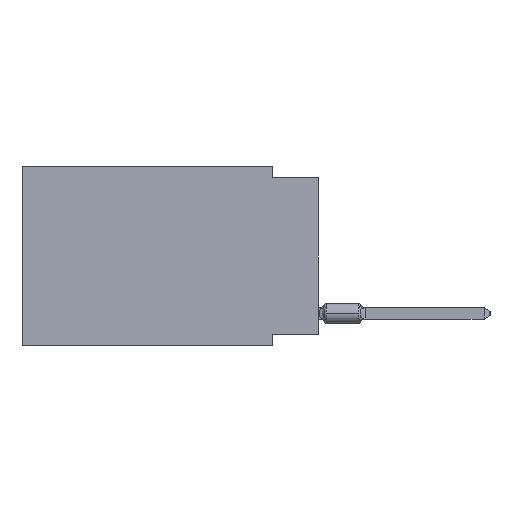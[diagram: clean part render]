
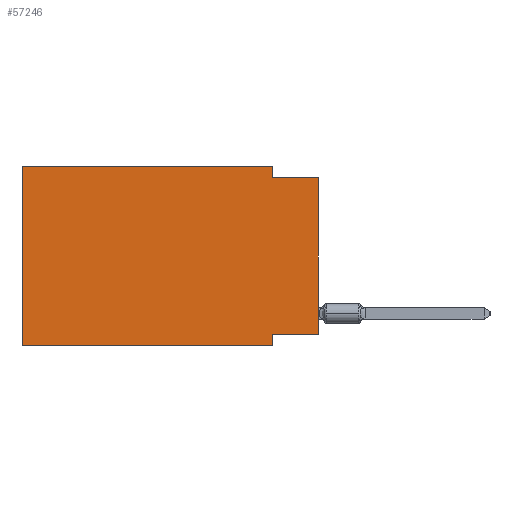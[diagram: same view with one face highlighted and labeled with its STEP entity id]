
A CAD part, left-side view. The second image highlights one B-rep face of the part: STEP entity #57246.
In plain terms, the highlighted planar face has unit normal (-1, 0, 0).
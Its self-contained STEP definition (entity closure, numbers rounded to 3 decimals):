
#86787 = CARTESIAN_POINT ( 'NONE',  ( 0., 0., -9.271 ) ) ;
#5160 = VERTEX_POINT ( 'NONE', #24850 ) ;
#6858 = VECTOR ( 'NONE', #38476, 1000. ) ;
#7060 = DIRECTION ( 'NONE',  ( 0., 0., 1. ) ) ;
#8186 = VERTEX_POINT ( 'NONE', #38046 ) ;
#8609 = ORIENTED_EDGE ( 'NONE', *, *, #69408, .F. ) ;
#11351 = CARTESIAN_POINT ( 'NONE',  ( 0., 0., -9.271 ) ) ;
#11446 = DIRECTION ( 'NONE',  ( 0., 0., 1. ) ) ;
#14628 = CARTESIAN_POINT ( 'NONE',  ( 0., 2.54, -9.906 ) ) ;
#14784 = ORIENTED_EDGE ( 'NONE', *, *, #72777, .F. ) ;
#16888 = CARTESIAN_POINT ( 'NONE',  ( 0., 0., -0.635 ) ) ;
#17199 = ORIENTED_EDGE ( 'NONE', *, *, #70519, .F. ) ;
#18508 = VECTOR ( 'NONE', #49311, 1000. ) ;
#19639 = AXIS2_PLACEMENT_3D ( 'NONE', #23659, #29806, #35949 ) ;
#22567 = CARTESIAN_POINT ( 'NONE',  ( 0., 2.54, 0. ) ) ;
#23274 = EDGE_CURVE ( 'NONE', #79118, #34935, #83549, .T. ) ;
#23659 = CARTESIAN_POINT ( 'NONE',  ( 0., 16.383, 0. ) ) ;
#24605 = CARTESIAN_POINT ( 'NONE',  ( 0., 16.383, 0. ) ) ;
#24850 = CARTESIAN_POINT ( 'NONE',  ( 0., 2.54, 0. ) ) ;
#26623 = LINE ( 'NONE', #59524, #39153 ) ;
#27717 = ORIENTED_EDGE ( 'NONE', *, *, #67584, .F. ) ;
#27816 = CARTESIAN_POINT ( 'NONE',  ( 0., 2.54, -9.906 ) ) ;
#29372 = PLANE ( 'NONE',  #19639 ) ;
#29806 = DIRECTION ( 'NONE',  ( 1., 0., 0. ) ) ;
#30338 = VERTEX_POINT ( 'NONE', #43389 ) ;
#33140 = EDGE_CURVE ( 'NONE', #37058, #34935, #53127, .T. ) ;
#34922 = LINE ( 'NONE', #54673, #37143 ) ;
#34935 = VERTEX_POINT ( 'NONE', #52392 ) ;
#35949 = DIRECTION ( 'NONE',  ( 0., 0., -1. ) ) ;
#37058 = VERTEX_POINT ( 'NONE', #86787 ) ;
#37143 = VECTOR ( 'NONE', #40199, 1000. ) ;
#37484 = DIRECTION ( 'NONE',  ( 0., -1., 0. ) ) ;
#38046 = CARTESIAN_POINT ( 'NONE',  ( 0., 16.383, -9.906 ) ) ;
#38190 = LINE ( 'NONE', #24605, #71627 ) ;
#38476 = DIRECTION ( 'NONE',  ( 0., 0., -1. ) ) ;
#38957 = LINE ( 'NONE', #11351, #84373 ) ;
#39153 = VECTOR ( 'NONE', #47222, 1000. ) ;
#40199 = DIRECTION ( 'NONE',  ( 0., -1., 0. ) ) ;
#42135 = VERTEX_POINT ( 'NONE', #14628 ) ;
#43389 = CARTESIAN_POINT ( 'NONE',  ( 0., 16.383, 0. ) ) ;
#45489 = LINE ( 'NONE', #27816, #6858 ) ;
#46971 = CARTESIAN_POINT ( 'NONE',  ( 0., 0., 0. ) ) ;
#47222 = DIRECTION ( 'NONE',  ( 0., -1., 0. ) ) ;
#48088 = VERTEX_POINT ( 'NONE', #66790 ) ;
#49311 = DIRECTION ( 'NONE',  ( 0., 0., -1. ) ) ;
#51524 = ORIENTED_EDGE ( 'NONE', *, *, #23274, .F. ) ;
#52392 = CARTESIAN_POINT ( 'NONE',  ( 0., 0., -0.635 ) ) ;
#53127 = LINE ( 'NONE', #46971, #82672 ) ;
#54673 = CARTESIAN_POINT ( 'NONE',  ( 0., 16.383, 0. ) ) ;
#55337 = ORIENTED_EDGE ( 'NONE', *, *, #79723, .T. ) ;
#57246 = ADVANCED_FACE ( 'NONE', ( #76295 ), #29372, .F. ) ;
#59524 = CARTESIAN_POINT ( 'NONE',  ( 0., 16.383, -9.906 ) ) ;
#66790 = CARTESIAN_POINT ( 'NONE',  ( 0., 2.54, -9.271 ) ) ;
#67584 = EDGE_CURVE ( 'NONE', #48088, #42135, #45489, .T. ) ;
#69408 = EDGE_CURVE ( 'NONE', #8186, #30338, #38190, .T. ) ;
#69538 = ORIENTED_EDGE ( 'NONE', *, *, #76524, .F. ) ;
#70519 = EDGE_CURVE ( 'NONE', #5160, #79118, #82654, .T. ) ;
#71627 = VECTOR ( 'NONE', #11446, 1000. ) ;
#72777 = EDGE_CURVE ( 'NONE', #37058, #48088, #38957, .T. ) ;
#73156 = VECTOR ( 'NONE', #37484, 1000. ) ;
#76295 = FACE_OUTER_BOUND ( 'NONE', #79788, .T. ) ;
#76524 = EDGE_CURVE ( 'NONE', #30338, #5160, #34922, .T. ) ;
#78025 = DIRECTION ( 'NONE',  ( 0., 1., 0. ) ) ;
#78928 = ORIENTED_EDGE ( 'NONE', *, *, #33140, .T. ) ;
#79118 = VERTEX_POINT ( 'NONE', #81311 ) ;
#79723 = EDGE_CURVE ( 'NONE', #8186, #42135, #26623, .T. ) ;
#79788 = EDGE_LOOP ( 'NONE', ( #78928, #51524, #17199, #69538, #8609, #55337, #27717, #14784 ) ) ;
#81311 = CARTESIAN_POINT ( 'NONE',  ( 0., 2.54, -0.635 ) ) ;
#82654 = LINE ( 'NONE', #22567, #18508 ) ;
#82672 = VECTOR ( 'NONE', #7060, 1000. ) ;
#83549 = LINE ( 'NONE', #16888, #73156 ) ;
#84373 = VECTOR ( 'NONE', #78025, 1000. ) ;
